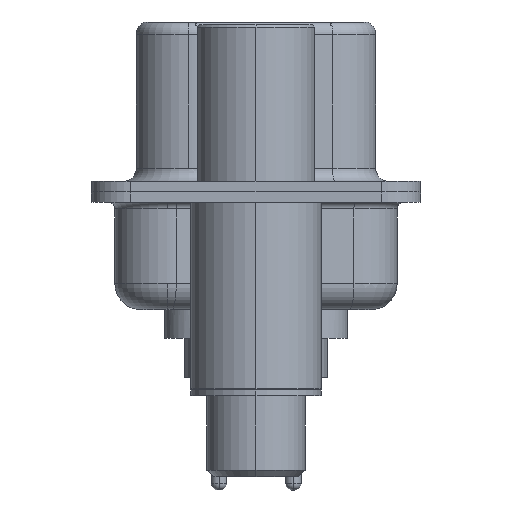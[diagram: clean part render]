
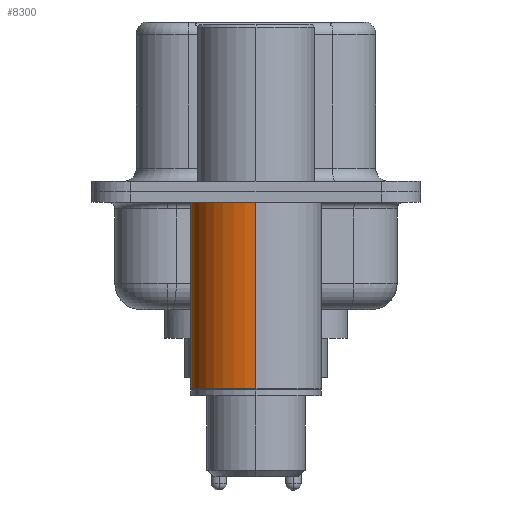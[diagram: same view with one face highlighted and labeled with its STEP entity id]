
A CAD part, left-side view. The second image highlights one B-rep face of the part: STEP entity #8300.
In plain terms, the highlighted cylindrical face has radius 2.5 mm (diameter 5 mm), a partial arc.
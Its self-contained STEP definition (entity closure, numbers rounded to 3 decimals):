
#1656 = EDGE_CURVE ( 'NONE', #14903, #7669, #20160, .T. ) ;
#2734 = VERTEX_POINT ( 'NONE', #19473 ) ;
#3982 = ORIENTED_EDGE ( 'NONE', *, *, #4797, .T. ) ;
#4794 = AXIS2_PLACEMENT_3D ( 'NONE', #22741, #8682, #25053 ) ;
#4797 = EDGE_CURVE ( 'NONE', #7669, #2734, #17387, .T. ) ;
#7213 = DIRECTION ( 'NONE',  ( 0., 0., 1. ) ) ;
#7257 = EDGE_LOOP ( 'NONE', ( #16327, #3982, #16498, #7960 ) ) ;
#7669 = VERTEX_POINT ( 'NONE', #14635 ) ;
#7960 = ORIENTED_EDGE ( 'NONE', *, *, #23825, .F. ) ;
#8300 = ADVANCED_FACE ( 'NONE', ( #19119 ), #17651, .T. ) ;
#8682 = DIRECTION ( 'NONE',  ( 0., 0., 1. ) ) ;
#9873 = CARTESIAN_POINT ( 'NONE',  ( 2.5, 0., -7.525 ) ) ;
#10377 = AXIS2_PLACEMENT_3D ( 'NONE', #24813, #24938, #24914 ) ;
#14173 = CARTESIAN_POINT ( 'NONE',  ( 2.5, 0., -0.4 ) ) ;
#14635 = CARTESIAN_POINT ( 'NONE',  ( -2.5, 0., -7.525 ) ) ;
#14903 = VERTEX_POINT ( 'NONE', #9873 ) ;
#16327 = ORIENTED_EDGE ( 'NONE', *, *, #1656, .T. ) ;
#16498 = ORIENTED_EDGE ( 'NONE', *, *, #29911, .F. ) ;
#16637 = VECTOR ( 'NONE', #7213, 1000. ) ;
#16696 = VERTEX_POINT ( 'NONE', #14173 ) ;
#17387 = LINE ( 'NONE', #18058, #16637 ) ;
#17651 = CYLINDRICAL_SURFACE ( 'NONE', #28942, 2.5 ) ;
#18058 = CARTESIAN_POINT ( 'NONE',  ( -2.5, 0., 0.581 ) ) ;
#18334 = CARTESIAN_POINT ( 'NONE',  ( 0., 0., 0.581 ) ) ;
#19119 = FACE_OUTER_BOUND ( 'NONE', #7257, .T. ) ;
#19473 = CARTESIAN_POINT ( 'NONE',  ( -2.5, 0., -0.4 ) ) ;
#20160 = CIRCLE ( 'NONE', #10377, 2.5 ) ;
#20602 = DIRECTION ( 'NONE',  ( 1., 0., 0. ) ) ;
#21925 = CARTESIAN_POINT ( 'NONE',  ( 2.5, 0., 0.581 ) ) ;
#22741 = CARTESIAN_POINT ( 'NONE',  ( 0., 0., -0.4 ) ) ;
#23010 = DIRECTION ( 'NONE',  ( 0., 0., 1. ) ) ;
#23211 = CIRCLE ( 'NONE', #4794, 2.5 ) ;
#23387 = VECTOR ( 'NONE', #24233, 1000. ) ;
#23825 = EDGE_CURVE ( 'NONE', #14903, #16696, #28805, .T. ) ;
#24233 = DIRECTION ( 'NONE',  ( 0., 0., 1. ) ) ;
#24813 = CARTESIAN_POINT ( 'NONE',  ( 0., 0., -7.525 ) ) ;
#24914 = DIRECTION ( 'NONE',  ( 1., 0., 0. ) ) ;
#24938 = DIRECTION ( 'NONE',  ( 0., 0., 1. ) ) ;
#25053 = DIRECTION ( 'NONE',  ( 1., 0., 0. ) ) ;
#28805 = LINE ( 'NONE', #21925, #23387 ) ;
#28942 = AXIS2_PLACEMENT_3D ( 'NONE', #18334, #23010, #20602 ) ;
#29911 = EDGE_CURVE ( 'NONE', #16696, #2734, #23211, .T. ) ;
